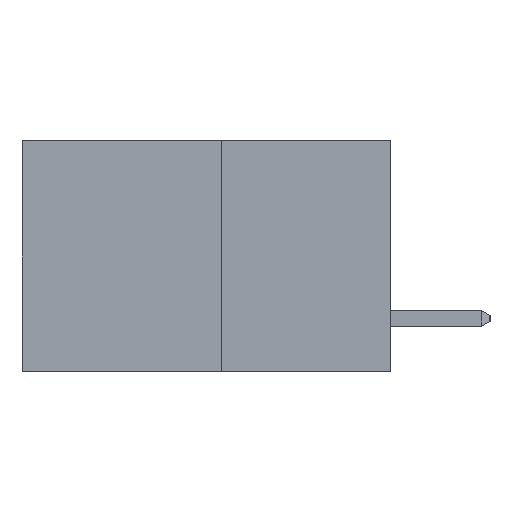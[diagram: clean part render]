
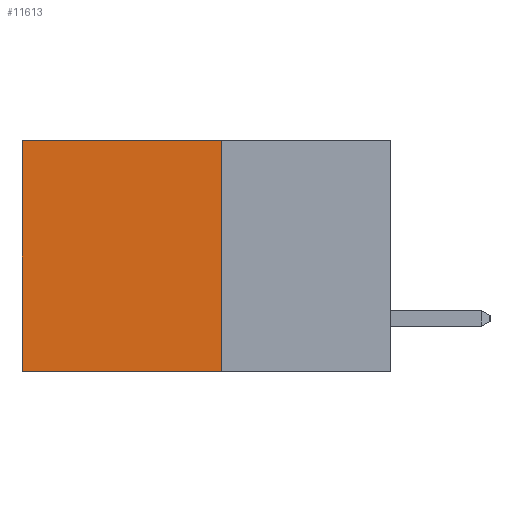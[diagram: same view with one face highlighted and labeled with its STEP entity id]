
A CAD part, left-side view. The second image highlights one B-rep face of the part: STEP entity #11613.
In plain terms, the highlighted planar face has unit normal (-1, 0, 0).
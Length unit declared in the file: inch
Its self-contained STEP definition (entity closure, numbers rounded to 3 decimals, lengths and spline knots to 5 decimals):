
#815 = CARTESIAN_POINT ( 'NONE',  ( 0.277, 0.27, 0. ) ) ;
#1118 = CARTESIAN_POINT ( 'NONE',  ( 0.277, 0.27, -0.37 ) ) ;
#1299 = ORIENTED_EDGE ( 'NONE', *, *, #8427, .F. ) ;
#1592 = DIRECTION ( 'NONE',  ( 1., 0., 0. ) ) ;
#1700 = FACE_OUTER_BOUND ( 'NONE', #3173, .T. ) ;
#2504 = DIRECTION ( 'NONE',  ( 0., 0., -1. ) ) ;
#2648 = LINE ( 'NONE', #815, #12099 ) ;
#3099 = LINE ( 'NONE', #1118, #13312 ) ;
#3173 = EDGE_LOOP ( 'NONE', ( #3239, #14207, #1299, #8353 ) ) ;
#3239 = ORIENTED_EDGE ( 'NONE', *, *, #14030, .T. ) ;
#3551 = DIRECTION ( 'NONE',  ( 0., 1., 0. ) ) ;
#3760 = EDGE_CURVE ( 'NONE', #12454, #11960, #13472, .T. ) ;
#3882 = LINE ( 'NONE', #5878, #13653 ) ;
#5878 = CARTESIAN_POINT ( 'NONE',  ( 0.277, 0.59, -0.37 ) ) ;
#6483 = CARTESIAN_POINT ( 'NONE',  ( 0.277, 0.59, 0. ) ) ;
#7184 = VERTEX_POINT ( 'NONE', #6483 ) ;
#8353 = ORIENTED_EDGE ( 'NONE', *, *, #8890, .T. ) ;
#8427 = EDGE_CURVE ( 'NONE', #12322, #12454, #3099, .T. ) ;
#8890 = EDGE_CURVE ( 'NONE', #12322, #7184, #2648, .T. ) ;
#9448 = CARTESIAN_POINT ( 'NONE',  ( 0.277, 0.27, -0.37 ) ) ;
#10698 = DIRECTION ( 'NONE',  ( 0., 0., -1. ) ) ;
#10852 = CARTESIAN_POINT ( 'NONE',  ( 0.277, 0.27, 0. ) ) ;
#11613 = ADVANCED_FACE ( 'NONE', ( #1700 ), #14424, .F. ) ;
#11895 = CARTESIAN_POINT ( 'NONE',  ( 0.277, 0.27, -0.37 ) ) ;
#11960 = VERTEX_POINT ( 'NONE', #16442 ) ;
#12099 = VECTOR ( 'NONE', #3551, 39.37008 ) ;
#12322 = VERTEX_POINT ( 'NONE', #10852 ) ;
#12454 = VERTEX_POINT ( 'NONE', #14882 ) ;
#13081 = VECTOR ( 'NONE', #15791, 39.37008 ) ;
#13312 = VECTOR ( 'NONE', #2504, 39.37008 ) ;
#13433 = DIRECTION ( 'NONE',  ( 0., 0., -1. ) ) ;
#13472 = LINE ( 'NONE', #11895, #13081 ) ;
#13636 = AXIS2_PLACEMENT_3D ( 'NONE', #9448, #1592, #10698 ) ;
#13653 = VECTOR ( 'NONE', #13433, 39.37008 ) ;
#14030 = EDGE_CURVE ( 'NONE', #7184, #11960, #3882, .T. ) ;
#14207 = ORIENTED_EDGE ( 'NONE', *, *, #3760, .F. ) ;
#14424 = PLANE ( 'NONE',  #13636 ) ;
#14882 = CARTESIAN_POINT ( 'NONE',  ( 0.277, 0.27, -0.37 ) ) ;
#15791 = DIRECTION ( 'NONE',  ( 0., 1., 0. ) ) ;
#16442 = CARTESIAN_POINT ( 'NONE',  ( 0.277, 0.59, -0.37 ) ) ;
